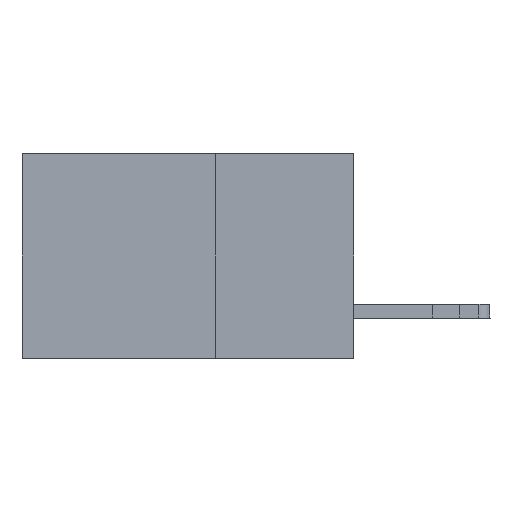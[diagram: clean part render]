
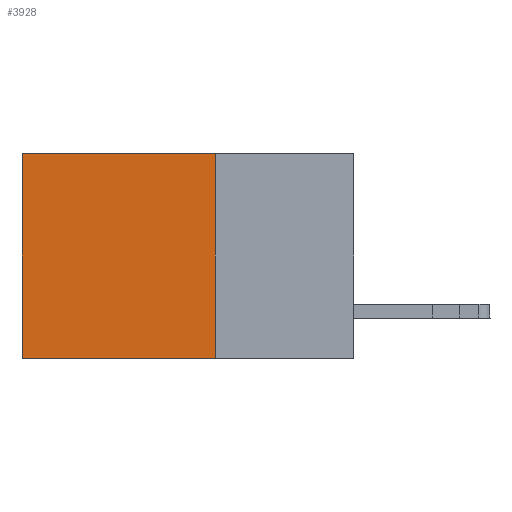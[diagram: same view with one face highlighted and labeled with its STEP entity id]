
A CAD part, left-side view. The second image highlights one B-rep face of the part: STEP entity #3928.
In plain terms, the highlighted planar face has unit normal (-1, 0, 0).
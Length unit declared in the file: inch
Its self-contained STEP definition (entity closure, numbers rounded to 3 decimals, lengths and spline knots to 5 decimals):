
#22 = ORIENTED_EDGE ( 'NONE', *, *, #7203, .T. ) ;
#225 = FACE_OUTER_BOUND ( 'NONE', #18402, .T. ) ;
#1549 = PLANE ( 'NONE',  #14396 ) ;
#1611 = DIRECTION ( 'NONE',  ( 1., 0., 0. ) ) ;
#1786 = CARTESIAN_POINT ( 'NONE',  ( 0.2875, 0.25, -0.37 ) ) ;
#2066 = CARTESIAN_POINT ( 'NONE',  ( 0.2875, 0.25, 0. ) ) ;
#3612 = VERTEX_POINT ( 'NONE', #5329 ) ;
#3730 = CARTESIAN_POINT ( 'NONE',  ( 0.2875, 0.25, -0.37 ) ) ;
#3928 = ADVANCED_FACE ( 'NONE', ( #225 ), #1549, .F. ) ;
#5329 = CARTESIAN_POINT ( 'NONE',  ( 0.2875, 0.6, 0. ) ) ;
#5442 = CARTESIAN_POINT ( 'NONE',  ( 0.2875, 0.6, 0. ) ) ;
#6929 = CARTESIAN_POINT ( 'NONE',  ( 0.2875, 0.25, 0. ) ) ;
#7147 = CARTESIAN_POINT ( 'NONE',  ( 0.2875, 0.6, -0.37 ) ) ;
#7203 = EDGE_CURVE ( 'NONE', #19378, #3612, #10417, .T. ) ;
#9109 = VECTOR ( 'NONE', #17793, 39.37008 ) ;
#9604 = DIRECTION ( 'NONE',  ( 0., 0., -1. ) ) ;
#10321 = CARTESIAN_POINT ( 'NONE',  ( 0.2875, 0.25, 0. ) ) ;
#10388 = DIRECTION ( 'NONE',  ( 0., 1., 0. ) ) ;
#10417 = LINE ( 'NONE', #6929, #19064 ) ;
#10850 = EDGE_CURVE ( 'NONE', #3612, #17394, #13515, .T. ) ;
#10888 = EDGE_CURVE ( 'NONE', #19378, #17350, #14047, .T. ) ;
#12036 = DIRECTION ( 'NONE',  ( 0., 0., -1. ) ) ;
#12334 = DIRECTION ( 'NONE',  ( 0., 0., -1. ) ) ;
#13515 = LINE ( 'NONE', #5442, #17542 ) ;
#14047 = LINE ( 'NONE', #2066, #18089 ) ;
#14396 = AXIS2_PLACEMENT_3D ( 'NONE', #20607, #1611, #12036 ) ;
#14879 = ORIENTED_EDGE ( 'NONE', *, *, #10850, .T. ) ;
#15444 = ORIENTED_EDGE ( 'NONE', *, *, #10888, .F. ) ;
#17350 = VERTEX_POINT ( 'NONE', #1786 ) ;
#17394 = VERTEX_POINT ( 'NONE', #7147 ) ;
#17542 = VECTOR ( 'NONE', #12334, 39.37008 ) ;
#17793 = DIRECTION ( 'NONE',  ( 0., 1., 0. ) ) ;
#18089 = VECTOR ( 'NONE', #9604, 39.37008 ) ;
#18402 = EDGE_LOOP ( 'NONE', ( #14879, #19083, #15444, #22 ) ) ;
#18556 = LINE ( 'NONE', #3730, #9109 ) ;
#19064 = VECTOR ( 'NONE', #10388, 39.37008 ) ;
#19083 = ORIENTED_EDGE ( 'NONE', *, *, #21225, .F. ) ;
#19378 = VERTEX_POINT ( 'NONE', #10321 ) ;
#20607 = CARTESIAN_POINT ( 'NONE',  ( 0.2875, 0.25, 0. ) ) ;
#21225 = EDGE_CURVE ( 'NONE', #17350, #17394, #18556, .T. ) ;
